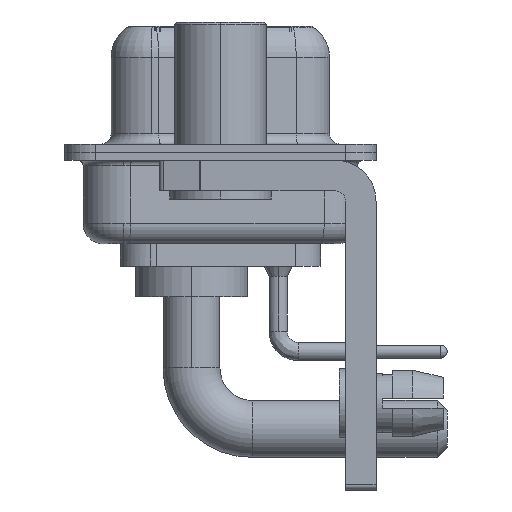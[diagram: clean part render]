
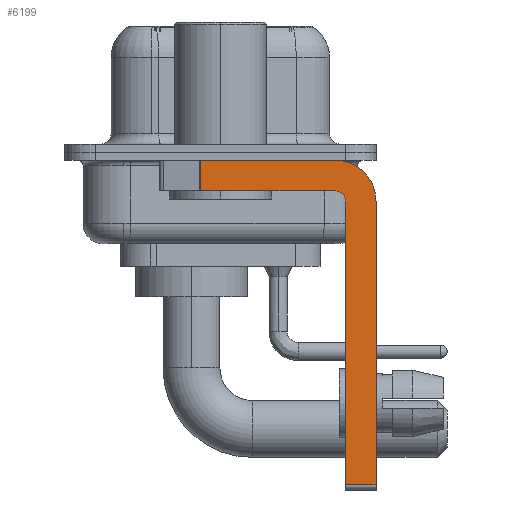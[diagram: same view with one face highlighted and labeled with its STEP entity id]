
A CAD part, left-side view. The second image highlights one B-rep face of the part: STEP entity #6199.
In plain terms, the highlighted planar face has unit normal (-1, 0, 0).
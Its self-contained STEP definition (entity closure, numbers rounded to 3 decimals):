
#165 = DIRECTION ( 'NONE',  ( 0., 0., -1. ) ) ;
#565 = CARTESIAN_POINT ( 'NONE',  ( -2.9, -7.65, -16.35 ) ) ;
#764 = VECTOR ( 'NONE', #13528, 1000. ) ;
#950 = EDGE_CURVE ( 'NONE', #15059, #18624, #16213, .T. ) ;
#1788 = VECTOR ( 'NONE', #165, 1000. ) ;
#1988 = CARTESIAN_POINT ( 'NONE',  ( -2.9, 0.978, -1.9 ) ) ;
#1999 = CARTESIAN_POINT ( 'NONE',  ( -2.9, -5.65, -2.4 ) ) ;
#2278 = EDGE_CURVE ( 'NONE', #14514, #13399, #7266, .T. ) ;
#2618 = VERTEX_POINT ( 'NONE', #22366 ) ;
#2646 = CARTESIAN_POINT ( 'NONE',  ( -2.9, -5.65, -2.4 ) ) ;
#2766 = CARTESIAN_POINT ( 'NONE',  ( -2.9, 3., -0.4 ) ) ;
#4434 = CARTESIAN_POINT ( 'NONE',  ( -2.9, -6.15, -2.4 ) ) ;
#4454 = DIRECTION ( 'NONE',  ( 0., 0., -1. ) ) ;
#4629 = DIRECTION ( 'NONE',  ( 1., 0., 0. ) ) ;
#4783 = ORIENTED_EDGE ( 'NONE', *, *, #12909, .F. ) ;
#5836 = DIRECTION ( 'NONE',  ( 0., 0., 1. ) ) ;
#5858 = EDGE_CURVE ( 'NONE', #7317, #13399, #23337, .T. ) ;
#6199 = ADVANCED_FACE ( 'NONE', ( #24482 ), #18449, .F. ) ;
#6803 = DIRECTION ( 'NONE',  ( 0., 0., -1. ) ) ;
#7266 = LINE ( 'NONE', #19168, #8627 ) ;
#7317 = VERTEX_POINT ( 'NONE', #16761 ) ;
#7541 = AXIS2_PLACEMENT_3D ( 'NONE', #24229, #4629, #6803 ) ;
#7795 = CARTESIAN_POINT ( 'NONE',  ( -2.9, -6.15, -16.6 ) ) ;
#8627 = VECTOR ( 'NONE', #11339, 1000. ) ;
#9246 = VERTEX_POINT ( 'NONE', #22818 ) ;
#9892 = ORIENTED_EDGE ( 'NONE', *, *, #950, .F. ) ;
#10814 = AXIS2_PLACEMENT_3D ( 'NONE', #1999, #11708, #5836 ) ;
#10976 = DIRECTION ( 'NONE',  ( 0., 1., 0. ) ) ;
#11134 = DIRECTION ( 'NONE',  ( 0., 0., -1. ) ) ;
#11339 = DIRECTION ( 'NONE',  ( 0., -1., 0. ) ) ;
#11470 = CARTESIAN_POINT ( 'NONE',  ( -2.9, -5.65, -1.9 ) ) ;
#11708 = DIRECTION ( 'NONE',  ( -1., 0., 0. ) ) ;
#12282 = EDGE_LOOP ( 'NONE', ( #9892, #21655, #24657, #15425, #4783, #23533, #15360, #24725 ) ) ;
#12479 = DIRECTION ( 'NONE',  ( 0., -1., 0. ) ) ;
#12526 = LINE ( 'NONE', #11470, #15004 ) ;
#12765 = CARTESIAN_POINT ( 'NONE',  ( -2.9, -6.15, -16.35 ) ) ;
#12909 = EDGE_CURVE ( 'NONE', #14514, #18158, #15457, .T. ) ;
#13399 = VERTEX_POINT ( 'NONE', #565 ) ;
#13528 = DIRECTION ( 'NONE',  ( 0., 0., 1. ) ) ;
#14230 = CARTESIAN_POINT ( 'NONE',  ( -2.9, -5.65, -0.4 ) ) ;
#14514 = VERTEX_POINT ( 'NONE', #12765 ) ;
#15004 = VECTOR ( 'NONE', #10976, 1000. ) ;
#15059 = VERTEX_POINT ( 'NONE', #19377 ) ;
#15255 = EDGE_CURVE ( 'NONE', #18624, #7317, #20157, .T. ) ;
#15360 = ORIENTED_EDGE ( 'NONE', *, *, #5858, .F. ) ;
#15425 = ORIENTED_EDGE ( 'NONE', *, *, #19113, .F. ) ;
#15457 = LINE ( 'NONE', #7795, #764 ) ;
#16213 = LINE ( 'NONE', #2766, #20749 ) ;
#16635 = EDGE_CURVE ( 'NONE', #15059, #2618, #17724, .T. ) ;
#16761 = CARTESIAN_POINT ( 'NONE',  ( -2.9, -7.65, -2.4 ) ) ;
#17724 = LINE ( 'NONE', #1988, #1788 ) ;
#18158 = VERTEX_POINT ( 'NONE', #4434 ) ;
#18449 = PLANE ( 'NONE',  #7541 ) ;
#18624 = VERTEX_POINT ( 'NONE', #14230 ) ;
#19113 = EDGE_CURVE ( 'NONE', #18158, #9246, #22280, .T. ) ;
#19168 = CARTESIAN_POINT ( 'NONE',  ( -2.9, -5.65, -16.35 ) ) ;
#19377 = CARTESIAN_POINT ( 'NONE',  ( -2.9, 0.978, -0.4 ) ) ;
#20061 = DIRECTION ( 'NONE',  ( 1., 0., 0. ) ) ;
#20157 = CIRCLE ( 'NONE', #21791, 2. ) ;
#20749 = VECTOR ( 'NONE', #12479, 1000. ) ;
#21655 = ORIENTED_EDGE ( 'NONE', *, *, #16635, .T. ) ;
#21791 = AXIS2_PLACEMENT_3D ( 'NONE', #2646, #20061, #4454 ) ;
#22280 = CIRCLE ( 'NONE', #10814, 0.5 ) ;
#22366 = CARTESIAN_POINT ( 'NONE',  ( -2.9, 0.978, -1.9 ) ) ;
#22818 = CARTESIAN_POINT ( 'NONE',  ( -2.9, -5.65, -1.9 ) ) ;
#23210 = EDGE_CURVE ( 'NONE', #9246, #2618, #12526, .T. ) ;
#23337 = LINE ( 'NONE', #25260, #24329 ) ;
#23533 = ORIENTED_EDGE ( 'NONE', *, *, #2278, .T. ) ;
#24229 = CARTESIAN_POINT ( 'NONE',  ( -2.9, -5.65, -2.4 ) ) ;
#24329 = VECTOR ( 'NONE', #11134, 1000. ) ;
#24482 = FACE_OUTER_BOUND ( 'NONE', #12282, .T. ) ;
#24657 = ORIENTED_EDGE ( 'NONE', *, *, #23210, .F. ) ;
#24725 = ORIENTED_EDGE ( 'NONE', *, *, #15255, .F. ) ;
#25260 = CARTESIAN_POINT ( 'NONE',  ( -2.9, -7.65, -2.4 ) ) ;
